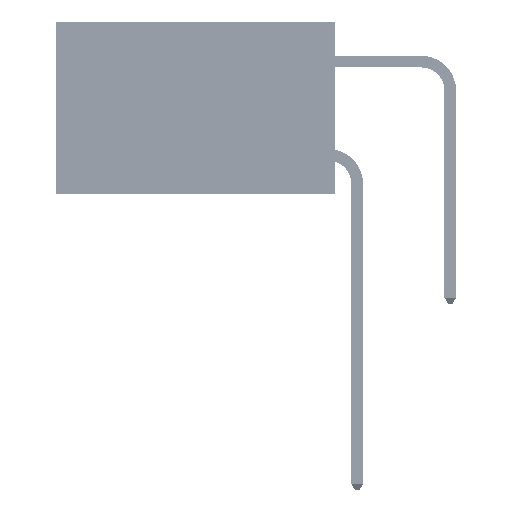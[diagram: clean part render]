
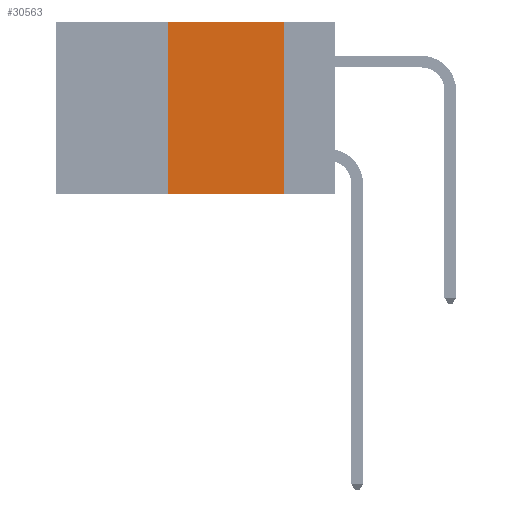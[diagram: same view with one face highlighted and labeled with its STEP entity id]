
A CAD part, left-side view. The second image highlights one B-rep face of the part: STEP entity #30563.
In plain terms, the highlighted planar face has unit normal (-1, 0, 0).
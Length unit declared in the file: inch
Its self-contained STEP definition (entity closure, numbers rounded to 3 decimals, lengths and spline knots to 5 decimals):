
#778 = LINE ( 'NONE', #31105, #46989 ) ;
#1192 = CARTESIAN_POINT ( 'NONE',  ( 0., 0.11, 0. ) ) ;
#1880 = DIRECTION ( 'NONE',  ( 0., 0., -1. ) ) ;
#2891 = LINE ( 'NONE', #1192, #34858 ) ;
#4564 = VECTOR ( 'NONE', #47837, 39.37008 ) ;
#7294 = FACE_OUTER_BOUND ( 'NONE', #21006, .T. ) ;
#8869 = LINE ( 'NONE', #18110, #35507 ) ;
#11494 = VERTEX_POINT ( 'NONE', #31630 ) ;
#12050 = ORIENTED_EDGE ( 'NONE', *, *, #47144, .F. ) ;
#12755 = CARTESIAN_POINT ( 'NONE',  ( 0., 0.36, -0.37 ) ) ;
#13179 = DIRECTION ( 'NONE',  ( 1., 0., 0. ) ) ;
#13602 = CARTESIAN_POINT ( 'NONE',  ( 0., 0.11, -0.37 ) ) ;
#14284 = VERTEX_POINT ( 'NONE', #42326 ) ;
#17940 = DIRECTION ( 'NONE',  ( 0., -1., 0. ) ) ;
#18110 = CARTESIAN_POINT ( 'NONE',  ( 0., 0.6, 0. ) ) ;
#20502 = EDGE_CURVE ( 'NONE', #33060, #22882, #27563, .T. ) ;
#21006 = EDGE_LOOP ( 'NONE', ( #25640, #43554, #12050, #28026 ) ) ;
#22882 = VERTEX_POINT ( 'NONE', #13602 ) ;
#23964 = DIRECTION ( 'NONE',  ( 0., 0., 1. ) ) ;
#24765 = AXIS2_PLACEMENT_3D ( 'NONE', #43578, #13179, #1880 ) ;
#25604 = CARTESIAN_POINT ( 'NONE',  ( 0., 0.6, -0.37 ) ) ;
#25640 = ORIENTED_EDGE ( 'NONE', *, *, #38003, .F. ) ;
#27563 = LINE ( 'NONE', #25604, #4564 ) ;
#28026 = ORIENTED_EDGE ( 'NONE', *, *, #20502, .T. ) ;
#30563 = ADVANCED_FACE ( 'NONE', ( #7294 ), #46893, .F. ) ;
#31105 = CARTESIAN_POINT ( 'NONE',  ( 0., 0.36, 0. ) ) ;
#31630 = CARTESIAN_POINT ( 'NONE',  ( 0., 0.11, 0. ) ) ;
#32779 = EDGE_CURVE ( 'NONE', #14284, #11494, #8869, .T. ) ;
#33060 = VERTEX_POINT ( 'NONE', #12755 ) ;
#34858 = VECTOR ( 'NONE', #38288, 39.37008 ) ;
#35507 = VECTOR ( 'NONE', #17940, 39.37008 ) ;
#38003 = EDGE_CURVE ( 'NONE', #11494, #22882, #2891, .T. ) ;
#38288 = DIRECTION ( 'NONE',  ( 0., 0., -1. ) ) ;
#42326 = CARTESIAN_POINT ( 'NONE',  ( 0., 0.36, 0. ) ) ;
#43554 = ORIENTED_EDGE ( 'NONE', *, *, #32779, .F. ) ;
#43578 = CARTESIAN_POINT ( 'NONE',  ( 0., 0.6, 0. ) ) ;
#46893 = PLANE ( 'NONE',  #24765 ) ;
#46989 = VECTOR ( 'NONE', #23964, 39.37008 ) ;
#47144 = EDGE_CURVE ( 'NONE', #33060, #14284, #778, .T. ) ;
#47837 = DIRECTION ( 'NONE',  ( 0., -1., 0. ) ) ;
